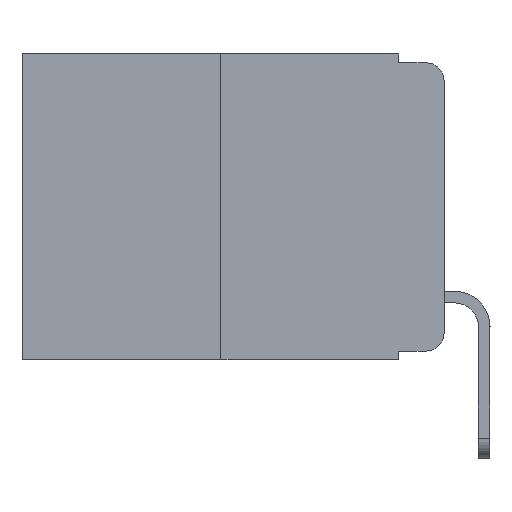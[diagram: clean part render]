
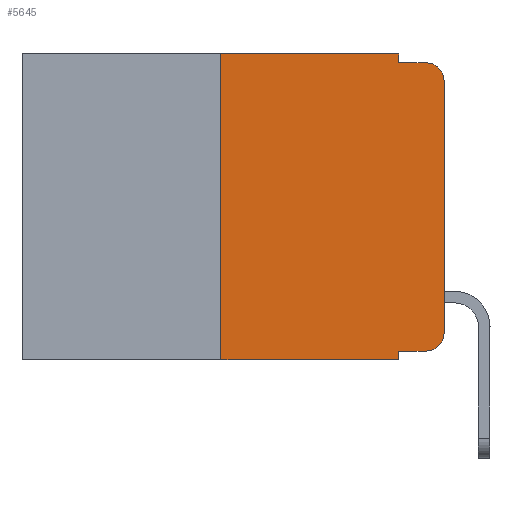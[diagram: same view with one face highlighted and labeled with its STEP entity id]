
A CAD part, left-side view. The second image highlights one B-rep face of the part: STEP entity #5645.
In plain terms, the highlighted planar face has unit normal (-1, 0, 0).
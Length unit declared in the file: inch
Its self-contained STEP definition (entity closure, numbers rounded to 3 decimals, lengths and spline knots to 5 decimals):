
#58 = CARTESIAN_POINT ( 'NONE',  ( 0., 0.051, -0.333 ) ) ;
#251 = EDGE_CURVE ( 'NONE', #2236, #3632, #1360, .T. ) ;
#995 = CARTESIAN_POINT ( 'NONE',  ( 0., 0.051, -0.333 ) ) ;
#1315 = DIRECTION ( 'NONE',  ( 0., 0., -1. ) ) ;
#1360 = CIRCLE ( 'NONE', #6781, 0.02 ) ;
#1472 = VECTOR ( 'NONE', #14363, 39.37008 ) ;
#1700 = DIRECTION ( 'NONE',  ( 1., 0., 0. ) ) ;
#1792 = CARTESIAN_POINT ( 'NONE',  ( 0., 0.051, 0. ) ) ;
#1901 = VERTEX_POINT ( 'NONE', #58 ) ;
#2225 = ORIENTED_EDGE ( 'NONE', *, *, #13263, .T. ) ;
#2236 = VERTEX_POINT ( 'NONE', #2645 ) ;
#2471 = ORIENTED_EDGE ( 'NONE', *, *, #6432, .T. ) ;
#2517 = CARTESIAN_POINT ( 'NONE',  ( 0., 0., -0.03 ) ) ;
#2645 = CARTESIAN_POINT ( 'NONE',  ( 0., 0.02, -0.333 ) ) ;
#2695 = CARTESIAN_POINT ( 'NONE',  ( 0., 0.051, 0. ) ) ;
#3053 = DIRECTION ( 'NONE',  ( 0., 0., -1. ) ) ;
#3157 = VERTEX_POINT ( 'NONE', #2517 ) ;
#3493 = VECTOR ( 'NONE', #3693, 39.37008 ) ;
#3632 = VERTEX_POINT ( 'NONE', #14699 ) ;
#3649 = VERTEX_POINT ( 'NONE', #14455 ) ;
#3693 = DIRECTION ( 'NONE',  ( 0., -1., 0. ) ) ;
#3878 = VERTEX_POINT ( 'NONE', #9695 ) ;
#3891 = VECTOR ( 'NONE', #15071, 39.37008 ) ;
#3956 = CARTESIAN_POINT ( 'NONE',  ( 0., 0.02, -0.03 ) ) ;
#4124 = VECTOR ( 'NONE', #10426, 39.37008 ) ;
#4165 = EDGE_CURVE ( 'NONE', #11512, #16725, #11774, .T. ) ;
#4527 = EDGE_LOOP ( 'NONE', ( #5543, #2225, #13475, #8527, #5380, #9375, #2471, #13036, #12989, #11588 ) ) ;
#4622 = LINE ( 'NONE', #5818, #16544 ) ;
#4655 = LINE ( 'NONE', #9840, #3891 ) ;
#4948 = EDGE_CURVE ( 'NONE', #3878, #8940, #4622, .T. ) ;
#5380 = ORIENTED_EDGE ( 'NONE', *, *, #9580, .F. ) ;
#5543 = ORIENTED_EDGE ( 'NONE', *, *, #14488, .T. ) ;
#5645 = ADVANCED_FACE ( 'NONE', ( #14333 ), #9516, .F. ) ;
#5818 = CARTESIAN_POINT ( 'NONE',  ( 0., 0.25, 0. ) ) ;
#6345 = CARTESIAN_POINT ( 'NONE',  ( 0., 0., 0. ) ) ;
#6432 = EDGE_CURVE ( 'NONE', #3878, #12965, #15619, .T. ) ;
#6781 = AXIS2_PLACEMENT_3D ( 'NONE', #10917, #12092, #13522 ) ;
#7785 = DIRECTION ( 'NONE',  ( 0., 0., 1. ) ) ;
#8234 = CARTESIAN_POINT ( 'NONE',  ( 0., 0.051, 0. ) ) ;
#8316 = CARTESIAN_POINT ( 'NONE',  ( 0., 0.051, -0.343 ) ) ;
#8472 = AXIS2_PLACEMENT_3D ( 'NONE', #14667, #1700, #3053 ) ;
#8527 = ORIENTED_EDGE ( 'NONE', *, *, #4165, .F. ) ;
#8602 = CIRCLE ( 'NONE', #13987, 0.02 ) ;
#8940 = VERTEX_POINT ( 'NONE', #12536 ) ;
#9031 = EDGE_CURVE ( 'NONE', #16725, #3649, #4655, .T. ) ;
#9042 = CARTESIAN_POINT ( 'NONE',  ( 0., 0.473, -0.343 ) ) ;
#9146 = LINE ( 'NONE', #6345, #16443 ) ;
#9226 = DIRECTION ( 'NONE',  ( -1., 0., 0. ) ) ;
#9375 = ORIENTED_EDGE ( 'NONE', *, *, #4948, .F. ) ;
#9516 = PLANE ( 'NONE',  #8472 ) ;
#9580 = EDGE_CURVE ( 'NONE', #8940, #11512, #13081, .T. ) ;
#9695 = CARTESIAN_POINT ( 'NONE',  ( 0., 0.25, -0.343 ) ) ;
#9840 = CARTESIAN_POINT ( 'NONE',  ( 0., 0.051, -0.01 ) ) ;
#10426 = DIRECTION ( 'NONE',  ( 0., 0., -1. ) ) ;
#10847 = DIRECTION ( 'NONE',  ( 0., 0., -1. ) ) ;
#10917 = CARTESIAN_POINT ( 'NONE',  ( 0., 0.02, -0.313 ) ) ;
#11438 = LINE ( 'NONE', #995, #12160 ) ;
#11512 = VERTEX_POINT ( 'NONE', #1792 ) ;
#11588 = ORIENTED_EDGE ( 'NONE', *, *, #251, .T. ) ;
#11774 = LINE ( 'NONE', #2695, #4124 ) ;
#11848 = VECTOR ( 'NONE', #10847, 39.37008 ) ;
#12092 = DIRECTION ( 'NONE',  ( -1., 0., 0. ) ) ;
#12160 = VECTOR ( 'NONE', #12453, 39.37008 ) ;
#12453 = DIRECTION ( 'NONE',  ( 0., -1., 0. ) ) ;
#12536 = CARTESIAN_POINT ( 'NONE',  ( 0., 0.25, 0. ) ) ;
#12965 = VERTEX_POINT ( 'NONE', #8316 ) ;
#12968 = EDGE_CURVE ( 'NONE', #1901, #12965, #14815, .T. ) ;
#12989 = ORIENTED_EDGE ( 'NONE', *, *, #15628, .T. ) ;
#13036 = ORIENTED_EDGE ( 'NONE', *, *, #12968, .F. ) ;
#13081 = LINE ( 'NONE', #14523, #1472 ) ;
#13263 = EDGE_CURVE ( 'NONE', #3157, #3649, #8602, .T. ) ;
#13475 = ORIENTED_EDGE ( 'NONE', *, *, #9031, .F. ) ;
#13522 = DIRECTION ( 'NONE',  ( 0., 0., -1. ) ) ;
#13987 = AXIS2_PLACEMENT_3D ( 'NONE', #3956, #9226, #1315 ) ;
#14333 = FACE_OUTER_BOUND ( 'NONE', #4527, .T. ) ;
#14363 = DIRECTION ( 'NONE',  ( 0., -1., 0. ) ) ;
#14455 = CARTESIAN_POINT ( 'NONE',  ( 0., 0.02, -0.01 ) ) ;
#14488 = EDGE_CURVE ( 'NONE', #3632, #3157, #9146, .T. ) ;
#14523 = CARTESIAN_POINT ( 'NONE',  ( 0., 0.473, 0. ) ) ;
#14667 = CARTESIAN_POINT ( 'NONE',  ( 0., 0.473, 0. ) ) ;
#14699 = CARTESIAN_POINT ( 'NONE',  ( 0., 0., -0.313 ) ) ;
#14815 = LINE ( 'NONE', #8234, #11848 ) ;
#15071 = DIRECTION ( 'NONE',  ( 0., -1., 0. ) ) ;
#15273 = CARTESIAN_POINT ( 'NONE',  ( 0., 0.051, -0.01 ) ) ;
#15619 = LINE ( 'NONE', #9042, #3493 ) ;
#15628 = EDGE_CURVE ( 'NONE', #1901, #2236, #11438, .T. ) ;
#16134 = DIRECTION ( 'NONE',  ( 0., 0., 1. ) ) ;
#16443 = VECTOR ( 'NONE', #7785, 39.37008 ) ;
#16544 = VECTOR ( 'NONE', #16134, 39.37008 ) ;
#16725 = VERTEX_POINT ( 'NONE', #15273 ) ;
